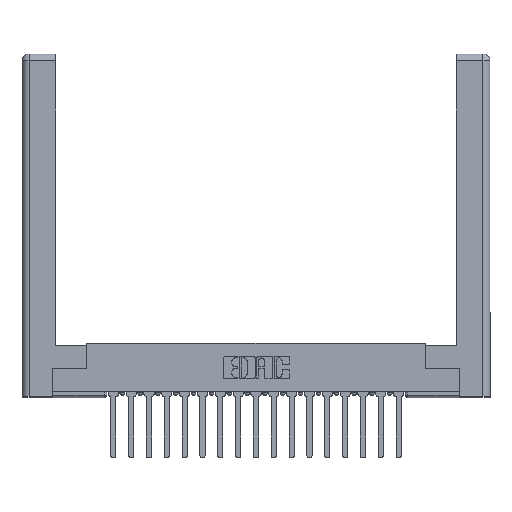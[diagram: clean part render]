
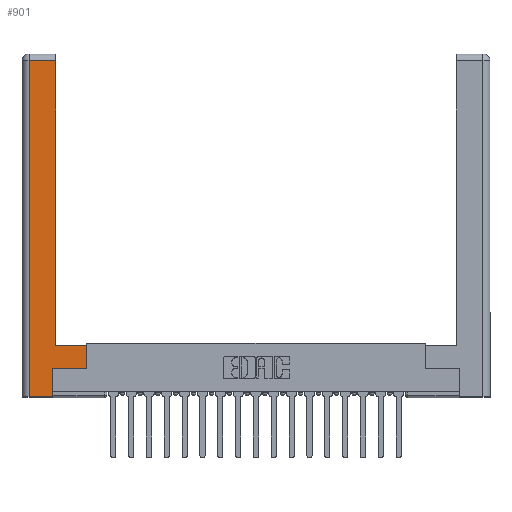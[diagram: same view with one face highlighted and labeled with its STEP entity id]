
A CAD part, top view. The second image highlights one B-rep face of the part: STEP entity #901.
In plain terms, the highlighted planar face has unit normal (0, 0, 1).
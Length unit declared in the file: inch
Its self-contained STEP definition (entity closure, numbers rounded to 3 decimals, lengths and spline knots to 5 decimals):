
#150 = VECTOR ( 'NONE', #572, 39.37008 ) ;
#572 = DIRECTION ( 'NONE',  ( 0., 1., 0. ) ) ;
#793 = CARTESIAN_POINT ( 'NONE',  ( 0.265, 0., 0. ) ) ;
#813 = ORIENTED_EDGE ( 'NONE', *, *, #3430, .T. ) ;
#901 = ADVANCED_FACE ( 'NONE', ( #16287 ), #16188, .F. ) ;
#1515 = VERTEX_POINT ( 'NONE', #13630 ) ;
#1817 = LINE ( 'NONE', #14491, #9451 ) ;
#1953 = CARTESIAN_POINT ( 'NONE',  ( 0.295, 0.45, 0. ) ) ;
#2066 = DIRECTION ( 'NONE',  ( 0., 0., -1. ) ) ;
#2440 = DIRECTION ( 'NONE',  ( 1., 0., 0. ) ) ;
#2544 = VERTEX_POINT ( 'NONE', #793 ) ;
#2555 = DIRECTION ( 'NONE',  ( 0., -1., 0. ) ) ;
#2813 = ORIENTED_EDGE ( 'NONE', *, *, #10868, .T. ) ;
#2927 = EDGE_CURVE ( 'NONE', #10544, #8185, #8991, .T. ) ;
#3430 = EDGE_CURVE ( 'NONE', #4710, #1515, #13602, .T. ) ;
#3534 = ORIENTED_EDGE ( 'NONE', *, *, #5587, .T. ) ;
#3817 = CARTESIAN_POINT ( 'NONE',  ( 0.565, 0.245, 0. ) ) ;
#4272 = EDGE_CURVE ( 'NONE', #1515, #13574, #13127, .T. ) ;
#4710 = VERTEX_POINT ( 'NONE', #16983 ) ;
#5480 = CARTESIAN_POINT ( 'NONE',  ( 0.0615, 2.94, 0. ) ) ;
#5587 = EDGE_CURVE ( 'NONE', #13574, #10344, #7034, .T. ) ;
#5909 = EDGE_CURVE ( 'NONE', #7605, #10544, #1817, .T. ) ;
#6357 = ORIENTED_EDGE ( 'NONE', *, *, #5909, .T. ) ;
#7034 = LINE ( 'NONE', #1953, #19057 ) ;
#7605 = VERTEX_POINT ( 'NONE', #8484 ) ;
#7980 = VECTOR ( 'NONE', #9566, 39.37008 ) ;
#8176 = CARTESIAN_POINT ( 'NONE',  ( 0., 0., 0. ) ) ;
#8185 = VERTEX_POINT ( 'NONE', #15786 ) ;
#8275 = DIRECTION ( 'NONE',  ( -1., 0., 0. ) ) ;
#8484 = CARTESIAN_POINT ( 'NONE',  ( 0.295, 2.94, 0. ) ) ;
#8503 = CARTESIAN_POINT ( 'NONE',  ( 0.565, 0.45, 0. ) ) ;
#8828 = DIRECTION ( 'NONE',  ( -1., 0., 0. ) ) ;
#8991 = LINE ( 'NONE', #16797, #9617 ) ;
#9078 = EDGE_CURVE ( 'NONE', #2544, #4710, #12068, .T. ) ;
#9451 = VECTOR ( 'NONE', #12888, 39.37008 ) ;
#9566 = DIRECTION ( 'NONE',  ( 1., 0., 0. ) ) ;
#9617 = VECTOR ( 'NONE', #2555, 39.37008 ) ;
#9885 = LINE ( 'NONE', #10102, #14198 ) ;
#9929 = ORIENTED_EDGE ( 'NONE', *, *, #2927, .T. ) ;
#9959 = AXIS2_PLACEMENT_3D ( 'NONE', #8176, #2066, #8275 ) ;
#10102 = CARTESIAN_POINT ( 'NONE',  ( 0.295, 3., 0. ) ) ;
#10344 = VERTEX_POINT ( 'NONE', #10391 ) ;
#10391 = CARTESIAN_POINT ( 'NONE',  ( 0.295, 0.45, 0. ) ) ;
#10544 = VERTEX_POINT ( 'NONE', #5480 ) ;
#10868 = EDGE_CURVE ( 'NONE', #8185, #2544, #12613, .T. ) ;
#11042 = CARTESIAN_POINT ( 'NONE',  ( 0.265, 0., 0. ) ) ;
#11557 = ORIENTED_EDGE ( 'NONE', *, *, #4272, .T. ) ;
#11958 = CARTESIAN_POINT ( 'NONE',  ( 0.265, 0.245, 0. ) ) ;
#12068 = LINE ( 'NONE', #11958, #150 ) ;
#12613 = LINE ( 'NONE', #11042, #7980 ) ;
#12888 = DIRECTION ( 'NONE',  ( -1., 0., 0. ) ) ;
#13127 = LINE ( 'NONE', #8503, #16042 ) ;
#13146 = ORIENTED_EDGE ( 'NONE', *, *, #14961, .T. ) ;
#13454 = DIRECTION ( 'NONE',  ( 0., 1., 0. ) ) ;
#13574 = VERTEX_POINT ( 'NONE', #14451 ) ;
#13602 = LINE ( 'NONE', #3817, #16698 ) ;
#13630 = CARTESIAN_POINT ( 'NONE',  ( 0.565, 0.245, 0. ) ) ;
#14198 = VECTOR ( 'NONE', #14732, 39.37008 ) ;
#14451 = CARTESIAN_POINT ( 'NONE',  ( 0.565, 0.45, 0. ) ) ;
#14491 = CARTESIAN_POINT ( 'NONE',  ( 0.0615, 2.94, 0. ) ) ;
#14732 = DIRECTION ( 'NONE',  ( 0., 1., 0. ) ) ;
#14961 = EDGE_CURVE ( 'NONE', #10344, #7605, #9885, .T. ) ;
#15582 = ORIENTED_EDGE ( 'NONE', *, *, #9078, .T. ) ;
#15786 = CARTESIAN_POINT ( 'NONE',  ( 0.0615, 0., 0. ) ) ;
#16042 = VECTOR ( 'NONE', #13454, 39.37008 ) ;
#16188 = PLANE ( 'NONE',  #9959 ) ;
#16287 = FACE_OUTER_BOUND ( 'NONE', #18143, .T. ) ;
#16698 = VECTOR ( 'NONE', #2440, 39.37008 ) ;
#16797 = CARTESIAN_POINT ( 'NONE',  ( 0.0615, 0., 0. ) ) ;
#16983 = CARTESIAN_POINT ( 'NONE',  ( 0.265, 0.245, 0. ) ) ;
#18143 = EDGE_LOOP ( 'NONE', ( #13146, #6357, #9929, #2813, #15582, #813, #11557, #3534 ) ) ;
#19057 = VECTOR ( 'NONE', #8828, 39.37008 ) ;
